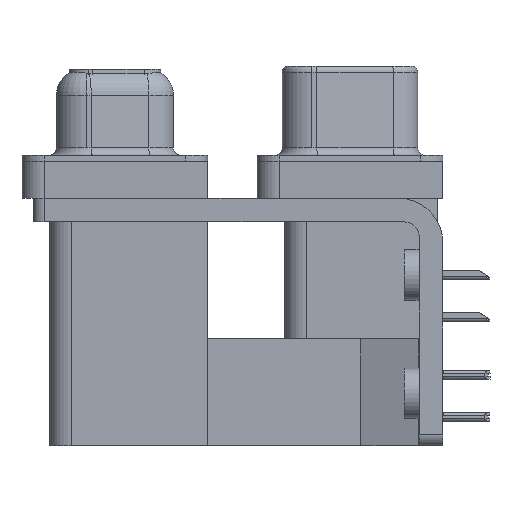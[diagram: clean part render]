
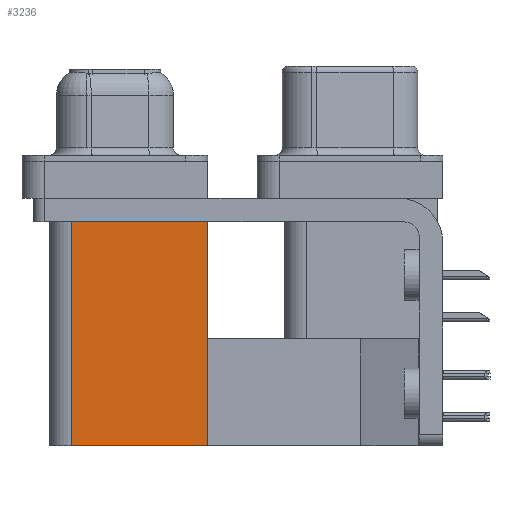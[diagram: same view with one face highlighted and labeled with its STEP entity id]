
A CAD part, left-side view. The second image highlights one B-rep face of the part: STEP entity #3236.
In plain terms, the highlighted planar face has unit normal (-1, 0, 0).
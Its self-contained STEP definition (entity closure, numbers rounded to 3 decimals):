
#447 = DIRECTION ( 'NONE',  ( 0., 0., 1. ) ) ;
#492 = CARTESIAN_POINT ( 'NONE',  ( 3.79, 9.6, -2.5 ) ) ;
#1952 = DIRECTION ( 'NONE',  ( 0., 1., 0. ) ) ;
#2944 = CARTESIAN_POINT ( 'NONE',  ( 3.79, 9.6, -19.2 ) ) ;
#3236 = ADVANCED_FACE ( 'NONE', ( #39143 ), #18639, .F. ) ;
#3530 = AXIS2_PLACEMENT_3D ( 'NONE', #26923, #11616, #36130 ) ;
#4187 = DIRECTION ( 'NONE',  ( 0., 0., 1. ) ) ;
#4520 = VERTEX_POINT ( 'NONE', #37633 ) ;
#4791 = VECTOR ( 'NONE', #1952, 1000. ) ;
#6109 = VERTEX_POINT ( 'NONE', #2944 ) ;
#6734 = ORIENTED_EDGE ( 'NONE', *, *, #7801, .F. ) ;
#7801 = EDGE_CURVE ( 'NONE', #6109, #4520, #11410, .T. ) ;
#9543 = VERTEX_POINT ( 'NONE', #16111 ) ;
#11123 = EDGE_LOOP ( 'NONE', ( #15000, #23412, #6734, #12641 ) ) ;
#11410 = LINE ( 'NONE', #32332, #4791 ) ;
#11616 = DIRECTION ( 'NONE',  ( 1., 0., 0. ) ) ;
#12072 = EDGE_CURVE ( 'NONE', #15313, #9543, #19620, .T. ) ;
#12641 = ORIENTED_EDGE ( 'NONE', *, *, #26033, .T. ) ;
#15000 = ORIENTED_EDGE ( 'NONE', *, *, #12072, .T. ) ;
#15313 = VERTEX_POINT ( 'NONE', #492 ) ;
#16111 = CARTESIAN_POINT ( 'NONE',  ( 3.79, 18.8, -2.5 ) ) ;
#17208 = CARTESIAN_POINT ( 'NONE',  ( 3.79, 9.6, -2.5 ) ) ;
#18639 = PLANE ( 'NONE',  #3530 ) ;
#19620 = LINE ( 'NONE', #17208, #28142 ) ;
#20071 = CARTESIAN_POINT ( 'NONE',  ( 3.79, 9.6, -19.2 ) ) ;
#20231 = DIRECTION ( 'NONE',  ( 0., 1., 0. ) ) ;
#20722 = VECTOR ( 'NONE', #4187, 1000. ) ;
#21786 = LINE ( 'NONE', #28801, #39186 ) ;
#22697 = LINE ( 'NONE', #20071, #20722 ) ;
#23412 = ORIENTED_EDGE ( 'NONE', *, *, #32865, .F. ) ;
#26033 = EDGE_CURVE ( 'NONE', #6109, #15313, #22697, .T. ) ;
#26923 = CARTESIAN_POINT ( 'NONE',  ( 3.79, 9.6, -19.2 ) ) ;
#28142 = VECTOR ( 'NONE', #20231, 1000. ) ;
#28801 = CARTESIAN_POINT ( 'NONE',  ( 3.79, 18.8, -19.2 ) ) ;
#32332 = CARTESIAN_POINT ( 'NONE',  ( 3.79, 9.6, -19.2 ) ) ;
#32865 = EDGE_CURVE ( 'NONE', #4520, #9543, #21786, .T. ) ;
#36130 = DIRECTION ( 'NONE',  ( 0., 1., 0. ) ) ;
#37633 = CARTESIAN_POINT ( 'NONE',  ( 3.79, 18.8, -19.2 ) ) ;
#39143 = FACE_OUTER_BOUND ( 'NONE', #11123, .T. ) ;
#39186 = VECTOR ( 'NONE', #447, 1000. ) ;
